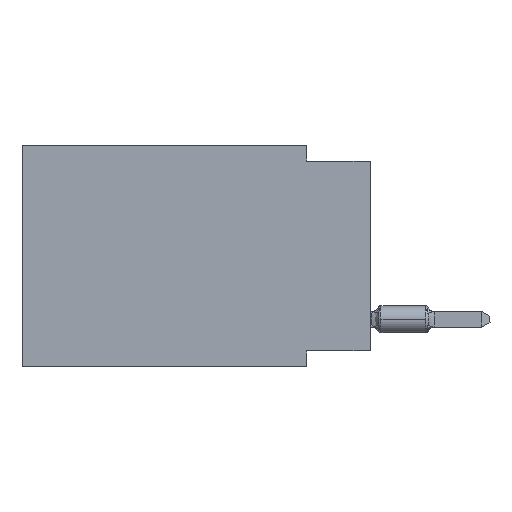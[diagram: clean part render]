
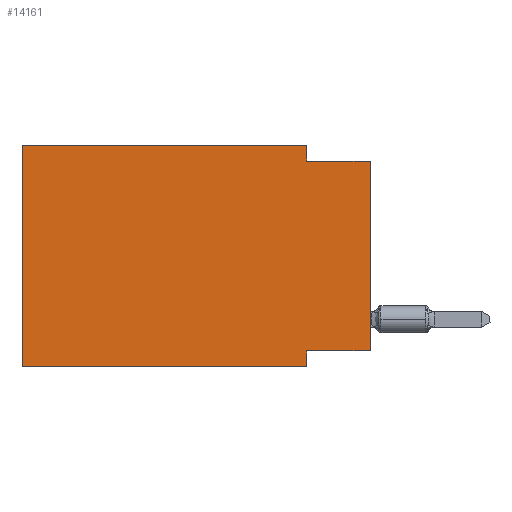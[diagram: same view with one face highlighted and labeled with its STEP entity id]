
A CAD part, left-side view. The second image highlights one B-rep face of the part: STEP entity #14161.
In plain terms, the highlighted planar face has unit normal (-1, 0, 0).
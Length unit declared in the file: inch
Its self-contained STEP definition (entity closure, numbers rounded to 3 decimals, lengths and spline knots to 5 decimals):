
#209 = VERTEX_POINT ( 'NONE', #14096 ) ;
#313 = LINE ( 'NONE', #7386, #10223 ) ;
#502 = EDGE_CURVE ( 'NONE', #8444, #6583, #1121, .T. ) ;
#604 = CARTESIAN_POINT ( 'NONE',  ( 0., 0., 0. ) ) ;
#787 = ORIENTED_EDGE ( 'NONE', *, *, #3403, .T. ) ;
#806 = EDGE_CURVE ( 'NONE', #11258, #10635, #3125, .T. ) ;
#997 = DIRECTION ( 'NONE',  ( 0., -1., 0. ) ) ;
#1121 = LINE ( 'NONE', #13451, #4962 ) ;
#1742 = AXIS2_PLACEMENT_3D ( 'NONE', #10191, #7594, #15360 ) ;
#1835 = CARTESIAN_POINT ( 'NONE',  ( 0., 0.1, -0.325 ) ) ;
#1948 = ORIENTED_EDGE ( 'NONE', *, *, #12981, .F. ) ;
#2197 = CARTESIAN_POINT ( 'NONE',  ( 0., 0.55, 0. ) ) ;
#2399 = LINE ( 'NONE', #4822, #11713 ) ;
#3125 = LINE ( 'NONE', #9401, #14723 ) ;
#3135 = CARTESIAN_POINT ( 'NONE',  ( 0., 0.1, -0.025 ) ) ;
#3403 = EDGE_CURVE ( 'NONE', #7668, #6583, #313, .T. ) ;
#3955 = CARTESIAN_POINT ( 'NONE',  ( 0., 0., -0.325 ) ) ;
#4094 = VECTOR ( 'NONE', #14699, 39.37008 ) ;
#4188 = LINE ( 'NONE', #3955, #4802 ) ;
#4356 = CARTESIAN_POINT ( 'NONE',  ( 0., 0., -0.025 ) ) ;
#4746 = EDGE_CURVE ( 'NONE', #209, #8444, #4188, .T. ) ;
#4802 = VECTOR ( 'NONE', #9132, 39.37008 ) ;
#4822 = CARTESIAN_POINT ( 'NONE',  ( 0., 0.55, 0. ) ) ;
#4962 = VECTOR ( 'NONE', #16820, 39.37008 ) ;
#4996 = CARTESIAN_POINT ( 'NONE',  ( 0., 0.1, -0.35 ) ) ;
#6039 = VECTOR ( 'NONE', #8133, 39.37008 ) ;
#6043 = ORIENTED_EDGE ( 'NONE', *, *, #4746, .F. ) ;
#6488 = CARTESIAN_POINT ( 'NONE',  ( 0., 0.1, 0. ) ) ;
#6583 = VERTEX_POINT ( 'NONE', #4996 ) ;
#7124 = ORIENTED_EDGE ( 'NONE', *, *, #10647, .T. ) ;
#7160 = EDGE_LOOP ( 'NONE', ( #7124, #13962, #1948, #12150, #8312, #787, #9102, #6043 ) ) ;
#7386 = CARTESIAN_POINT ( 'NONE',  ( 0., 0.55, -0.35 ) ) ;
#7418 = DIRECTION ( 'NONE',  ( 0., 0., 1. ) ) ;
#7515 = VERTEX_POINT ( 'NONE', #11453 ) ;
#7518 = LINE ( 'NONE', #604, #4094 ) ;
#7594 = DIRECTION ( 'NONE',  ( 1., 0., 0. ) ) ;
#7668 = VERTEX_POINT ( 'NONE', #13194 ) ;
#8039 = FACE_OUTER_BOUND ( 'NONE', #7160, .T. ) ;
#8133 = DIRECTION ( 'NONE',  ( 0., 0., -1. ) ) ;
#8312 = ORIENTED_EDGE ( 'NONE', *, *, #12842, .F. ) ;
#8444 = VERTEX_POINT ( 'NONE', #1835 ) ;
#9102 = ORIENTED_EDGE ( 'NONE', *, *, #502, .F. ) ;
#9132 = DIRECTION ( 'NONE',  ( 0., 1., 0. ) ) ;
#9401 = CARTESIAN_POINT ( 'NONE',  ( 0., 0., -0.025 ) ) ;
#10191 = CARTESIAN_POINT ( 'NONE',  ( 0., 0.55, 0. ) ) ;
#10223 = VECTOR ( 'NONE', #16272, 39.37008 ) ;
#10635 = VERTEX_POINT ( 'NONE', #4356 ) ;
#10647 = EDGE_CURVE ( 'NONE', #209, #10635, #7518, .T. ) ;
#10737 = VERTEX_POINT ( 'NONE', #16407 ) ;
#11258 = VERTEX_POINT ( 'NONE', #3135 ) ;
#11453 = CARTESIAN_POINT ( 'NONE',  ( 0., 0.1, 0. ) ) ;
#11577 = PLANE ( 'NONE',  #1742 ) ;
#11713 = VECTOR ( 'NONE', #7418, 39.37008 ) ;
#12150 = ORIENTED_EDGE ( 'NONE', *, *, #14036, .F. ) ;
#12842 = EDGE_CURVE ( 'NONE', #7668, #10737, #2399, .T. ) ;
#12981 = EDGE_CURVE ( 'NONE', #7515, #11258, #15406, .T. ) ;
#13194 = CARTESIAN_POINT ( 'NONE',  ( 0., 0.55, -0.35 ) ) ;
#13451 = CARTESIAN_POINT ( 'NONE',  ( 0., 0.1, -0.35 ) ) ;
#13962 = ORIENTED_EDGE ( 'NONE', *, *, #806, .F. ) ;
#14036 = EDGE_CURVE ( 'NONE', #10737, #7515, #15584, .T. ) ;
#14096 = CARTESIAN_POINT ( 'NONE',  ( 0., 0., -0.325 ) ) ;
#14161 = ADVANCED_FACE ( 'NONE', ( #8039 ), #11577, .F. ) ;
#14699 = DIRECTION ( 'NONE',  ( 0., 0., 1. ) ) ;
#14723 = VECTOR ( 'NONE', #16102, 39.37008 ) ;
#15360 = DIRECTION ( 'NONE',  ( 0., 0., -1. ) ) ;
#15399 = VECTOR ( 'NONE', #997, 39.37008 ) ;
#15406 = LINE ( 'NONE', #6488, #6039 ) ;
#15584 = LINE ( 'NONE', #2197, #15399 ) ;
#16102 = DIRECTION ( 'NONE',  ( 0., -1., 0. ) ) ;
#16272 = DIRECTION ( 'NONE',  ( 0., -1., 0. ) ) ;
#16407 = CARTESIAN_POINT ( 'NONE',  ( 0., 0.55, 0. ) ) ;
#16820 = DIRECTION ( 'NONE',  ( 0., 0., -1. ) ) ;
